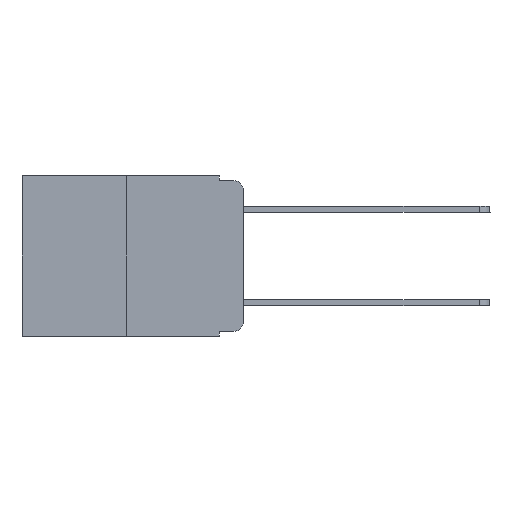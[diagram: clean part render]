
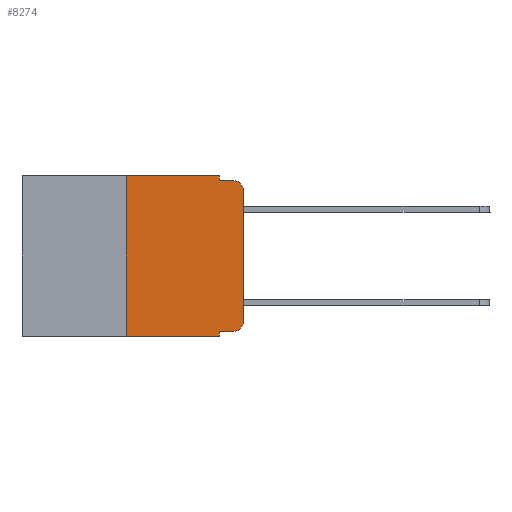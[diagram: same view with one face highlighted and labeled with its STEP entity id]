
A CAD part, left-side view. The second image highlights one B-rep face of the part: STEP entity #8274.
In plain terms, the highlighted planar face has unit normal (-1, 0, 0).
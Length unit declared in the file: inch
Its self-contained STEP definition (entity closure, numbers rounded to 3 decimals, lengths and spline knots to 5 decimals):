
#236 = VERTEX_POINT ( 'NONE', #10086 ) ;
#248 = VECTOR ( 'NONE', #14984, 39.37008 ) ;
#402 = ORIENTED_EDGE ( 'NONE', *, *, #15784, .T. ) ;
#617 = ORIENTED_EDGE ( 'NONE', *, *, #5847, .F. ) ;
#706 = LINE ( 'NONE', #6836, #5766 ) ;
#1157 = VERTEX_POINT ( 'NONE', #7085 ) ;
#1715 = EDGE_CURVE ( 'NONE', #8887, #2610, #706, .T. ) ;
#1737 = EDGE_CURVE ( 'NONE', #11962, #6827, #14315, .T. ) ;
#2610 = VERTEX_POINT ( 'NONE', #16342 ) ;
#2951 = DIRECTION ( 'NONE',  ( -1., 0., 0. ) ) ;
#2968 = DIRECTION ( 'NONE',  ( 1., 0., 0. ) ) ;
#3092 = ORIENTED_EDGE ( 'NONE', *, *, #4342, .T. ) ;
#3257 = CARTESIAN_POINT ( 'NONE',  ( 0., 0.051, -0.01 ) ) ;
#3273 = EDGE_CURVE ( 'NONE', #13016, #236, #9021, .T. ) ;
#3996 = DIRECTION ( 'NONE',  ( 0., 0., -1. ) ) ;
#4058 = DIRECTION ( 'NONE',  ( 0., -1., 0. ) ) ;
#4077 = ORIENTED_EDGE ( 'NONE', *, *, #5415, .T. ) ;
#4342 = EDGE_CURVE ( 'NONE', #2610, #236, #4812, .T. ) ;
#4812 = CIRCLE ( 'NONE', #14823, 0.02 ) ;
#5415 = EDGE_CURVE ( 'NONE', #6827, #8887, #11381, .T. ) ;
#5747 = VERTEX_POINT ( 'NONE', #17914 ) ;
#5766 = VECTOR ( 'NONE', #6781, 39.37008 ) ;
#5847 = EDGE_CURVE ( 'NONE', #10445, #13016, #11774, .T. ) ;
#5886 = VERTEX_POINT ( 'NONE', #12219 ) ;
#5911 = DIRECTION ( 'NONE',  ( 0., -1., 0. ) ) ;
#6004 = DIRECTION ( 'NONE',  ( 0., 0., -1. ) ) ;
#6120 = DIRECTION ( 'NONE',  ( -1., 0., 0. ) ) ;
#6395 = VECTOR ( 'NONE', #3996, 39.37008 ) ;
#6781 = DIRECTION ( 'NONE',  ( 0., 0., 1. ) ) ;
#6827 = VERTEX_POINT ( 'NONE', #12726 ) ;
#6836 = CARTESIAN_POINT ( 'NONE',  ( 0., 0., 0. ) ) ;
#6914 = VECTOR ( 'NONE', #4058, 39.37008 ) ;
#6992 = CARTESIAN_POINT ( 'NONE',  ( 0., 0.051, 0. ) ) ;
#7085 = CARTESIAN_POINT ( 'NONE',  ( 0., 0.25, -0.343 ) ) ;
#7417 = ORIENTED_EDGE ( 'NONE', *, *, #3273, .F. ) ;
#7778 = CARTESIAN_POINT ( 'NONE',  ( 0., 0.051, -0.333 ) ) ;
#7809 = EDGE_LOOP ( 'NONE', ( #17187, #3092, #7417, #617, #11937, #10145, #402, #9921, #16589, #4077 ) ) ;
#8007 = VECTOR ( 'NONE', #5911, 39.37008 ) ;
#8274 = ADVANCED_FACE ( 'NONE', ( #8924 ), #15658, .F. ) ;
#8316 = CARTESIAN_POINT ( 'NONE',  ( 0., 0., -0.313 ) ) ;
#8548 = CARTESIAN_POINT ( 'NONE',  ( 0., 0.473, 0. ) ) ;
#8887 = VERTEX_POINT ( 'NONE', #8316 ) ;
#8924 = FACE_OUTER_BOUND ( 'NONE', #7809, .T. ) ;
#9021 = LINE ( 'NONE', #3257, #13432 ) ;
#9350 = AXIS2_PLACEMENT_3D ( 'NONE', #8548, #2968, #15776 ) ;
#9493 = DIRECTION ( 'NONE',  ( 0., -1., 0. ) ) ;
#9517 = CARTESIAN_POINT ( 'NONE',  ( 0., 0.051, 0. ) ) ;
#9648 = DIRECTION ( 'NONE',  ( 0., 0., -1. ) ) ;
#9796 = AXIS2_PLACEMENT_3D ( 'NONE', #15585, #2951, #12957 ) ;
#9921 = ORIENTED_EDGE ( 'NONE', *, *, #10922, .F. ) ;
#9959 = VECTOR ( 'NONE', #9493, 39.37008 ) ;
#10086 = CARTESIAN_POINT ( 'NONE',  ( 0., 0.02, -0.01 ) ) ;
#10145 = ORIENTED_EDGE ( 'NONE', *, *, #17930, .F. ) ;
#10445 = VERTEX_POINT ( 'NONE', #6992 ) ;
#10650 = LINE ( 'NONE', #16623, #6914 ) ;
#10922 = EDGE_CURVE ( 'NONE', #11962, #5747, #17585, .T. ) ;
#10926 = CARTESIAN_POINT ( 'NONE',  ( 0., 0.051, -0.01 ) ) ;
#11348 = VECTOR ( 'NONE', #9648, 39.37008 ) ;
#11381 = CIRCLE ( 'NONE', #9796, 0.02 ) ;
#11462 = CARTESIAN_POINT ( 'NONE',  ( 0., 0.473, -0.343 ) ) ;
#11774 = LINE ( 'NONE', #12339, #11348 ) ;
#11937 = ORIENTED_EDGE ( 'NONE', *, *, #15675, .F. ) ;
#11962 = VERTEX_POINT ( 'NONE', #7778 ) ;
#11991 = CARTESIAN_POINT ( 'NONE',  ( 0., 0.25, 0. ) ) ;
#12191 = LINE ( 'NONE', #11462, #8007 ) ;
#12219 = CARTESIAN_POINT ( 'NONE',  ( 0., 0.25, 0. ) ) ;
#12339 = CARTESIAN_POINT ( 'NONE',  ( 0., 0.051, 0. ) ) ;
#12726 = CARTESIAN_POINT ( 'NONE',  ( 0., 0.02, -0.333 ) ) ;
#12957 = DIRECTION ( 'NONE',  ( 0., 0., -1. ) ) ;
#13016 = VERTEX_POINT ( 'NONE', #10926 ) ;
#13103 = DIRECTION ( 'NONE',  ( 0., -1., 0. ) ) ;
#13432 = VECTOR ( 'NONE', #13103, 39.37008 ) ;
#14315 = LINE ( 'NONE', #16549, #9959 ) ;
#14413 = CARTESIAN_POINT ( 'NONE',  ( 0., 0.02, -0.03 ) ) ;
#14823 = AXIS2_PLACEMENT_3D ( 'NONE', #14413, #6120, #6004 ) ;
#14984 = DIRECTION ( 'NONE',  ( 0., 0., 1. ) ) ;
#15585 = CARTESIAN_POINT ( 'NONE',  ( 0., 0.02, -0.313 ) ) ;
#15658 = PLANE ( 'NONE',  #9350 ) ;
#15675 = EDGE_CURVE ( 'NONE', #5886, #10445, #10650, .T. ) ;
#15776 = DIRECTION ( 'NONE',  ( 0., 0., -1. ) ) ;
#15784 = EDGE_CURVE ( 'NONE', #1157, #5747, #12191, .T. ) ;
#16342 = CARTESIAN_POINT ( 'NONE',  ( 0., 0., -0.03 ) ) ;
#16549 = CARTESIAN_POINT ( 'NONE',  ( 0., 0.051, -0.333 ) ) ;
#16589 = ORIENTED_EDGE ( 'NONE', *, *, #1737, .T. ) ;
#16623 = CARTESIAN_POINT ( 'NONE',  ( 0., 0.473, 0. ) ) ;
#16732 = LINE ( 'NONE', #11991, #248 ) ;
#17187 = ORIENTED_EDGE ( 'NONE', *, *, #1715, .T. ) ;
#17585 = LINE ( 'NONE', #9517, #6395 ) ;
#17914 = CARTESIAN_POINT ( 'NONE',  ( 0., 0.051, -0.343 ) ) ;
#17930 = EDGE_CURVE ( 'NONE', #1157, #5886, #16732, .T. ) ;
